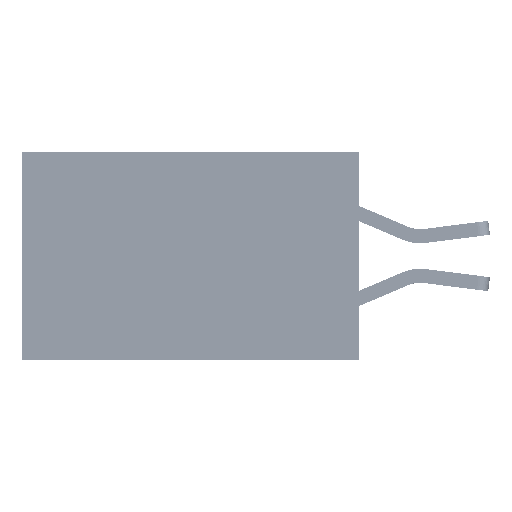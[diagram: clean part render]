
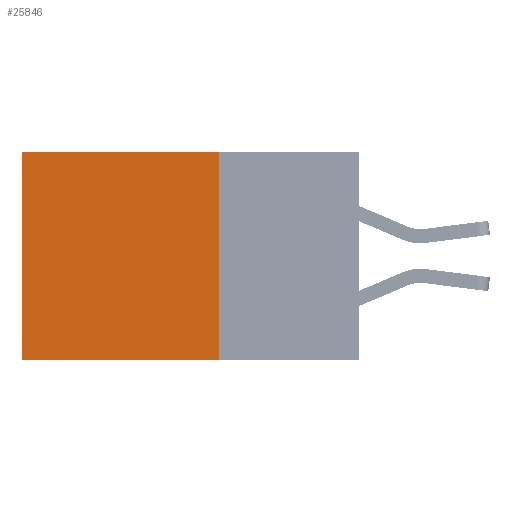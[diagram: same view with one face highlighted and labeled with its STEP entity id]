
A CAD part, left-side view. The second image highlights one B-rep face of the part: STEP entity #25846.
In plain terms, the highlighted planar face has unit normal (-1, 0, 0).
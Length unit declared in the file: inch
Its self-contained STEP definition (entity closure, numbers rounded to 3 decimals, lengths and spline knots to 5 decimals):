
#1406 = VERTEX_POINT ( 'NONE', #30348 ) ;
#3402 = EDGE_LOOP ( 'NONE', ( #41185, #42333, #31441, #30216 ) ) ;
#4033 = FACE_OUTER_BOUND ( 'NONE', #3402, .T. ) ;
#4128 = CARTESIAN_POINT ( 'NONE',  ( 0.2875, 0.25, 0. ) ) ;
#5927 = VERTEX_POINT ( 'NONE', #20554 ) ;
#6143 = DIRECTION ( 'NONE',  ( 0., 0., -1. ) ) ;
#10268 = LINE ( 'NONE', #47750, #47397 ) ;
#10539 = CARTESIAN_POINT ( 'NONE',  ( 0.2875, 0.6, -0.37 ) ) ;
#12344 = LINE ( 'NONE', #36312, #13542 ) ;
#13129 = AXIS2_PLACEMENT_3D ( 'NONE', #43367, #13560, #6143 ) ;
#13542 = VECTOR ( 'NONE', #13742, 39.37008 ) ;
#13560 = DIRECTION ( 'NONE',  ( 1., 0., 0. ) ) ;
#13742 = DIRECTION ( 'NONE',  ( 0., 0., -1. ) ) ;
#20554 = CARTESIAN_POINT ( 'NONE',  ( 0.2875, 0.25, -0.37 ) ) ;
#23518 = LINE ( 'NONE', #44335, #45880 ) ;
#24765 = PLANE ( 'NONE',  #13129 ) ;
#25846 = ADVANCED_FACE ( 'NONE', ( #4033 ), #24765, .F. ) ;
#27047 = DIRECTION ( 'NONE',  ( 0., 0., -1. ) ) ;
#28615 = LINE ( 'NONE', #4128, #39267 ) ;
#28943 = EDGE_CURVE ( 'NONE', #47878, #5927, #28615, .T. ) ;
#30216 = ORIENTED_EDGE ( 'NONE', *, *, #48167, .T. ) ;
#30348 = CARTESIAN_POINT ( 'NONE',  ( 0.2875, 0.6, 0. ) ) ;
#31321 = CARTESIAN_POINT ( 'NONE',  ( 0.2875, 0.25, 0. ) ) ;
#31441 = ORIENTED_EDGE ( 'NONE', *, *, #28943, .F. ) ;
#36293 = DIRECTION ( 'NONE',  ( 0., 1., 0. ) ) ;
#36312 = CARTESIAN_POINT ( 'NONE',  ( 0.2875, 0.6, 0. ) ) ;
#36403 = EDGE_CURVE ( 'NONE', #1406, #42649, #12344, .T. ) ;
#39267 = VECTOR ( 'NONE', #27047, 39.37008 ) ;
#41185 = ORIENTED_EDGE ( 'NONE', *, *, #36403, .T. ) ;
#42333 = ORIENTED_EDGE ( 'NONE', *, *, #45237, .F. ) ;
#42649 = VERTEX_POINT ( 'NONE', #10539 ) ;
#43367 = CARTESIAN_POINT ( 'NONE',  ( 0.2875, 0.25, 0. ) ) ;
#44335 = CARTESIAN_POINT ( 'NONE',  ( 0.2875, 0.25, -0.37 ) ) ;
#45237 = EDGE_CURVE ( 'NONE', #5927, #42649, #23518, .T. ) ;
#45880 = VECTOR ( 'NONE', #36293, 39.37008 ) ;
#47397 = VECTOR ( 'NONE', #47437, 39.37008 ) ;
#47437 = DIRECTION ( 'NONE',  ( 0., 1., 0. ) ) ;
#47750 = CARTESIAN_POINT ( 'NONE',  ( 0.2875, 0.25, 0. ) ) ;
#47878 = VERTEX_POINT ( 'NONE', #31321 ) ;
#48167 = EDGE_CURVE ( 'NONE', #47878, #1406, #10268, .T. ) ;
